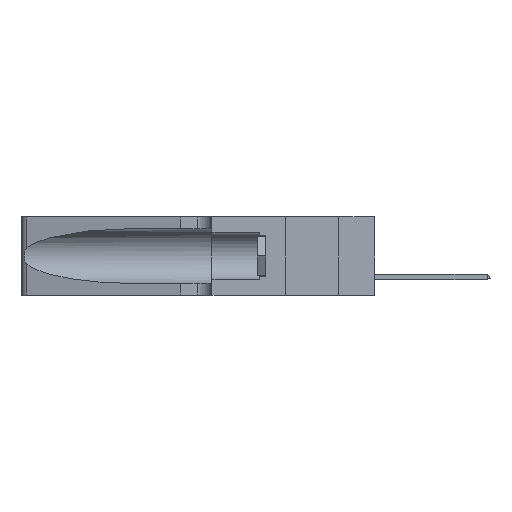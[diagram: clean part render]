
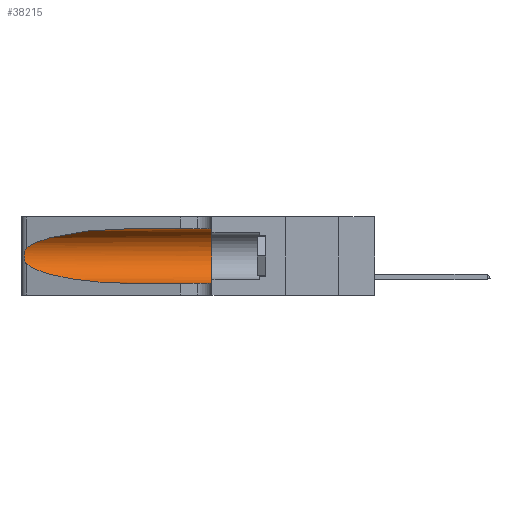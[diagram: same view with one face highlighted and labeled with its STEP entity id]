
A CAD part, left-side view. The second image highlights one B-rep face of the part: STEP entity #38215.
In plain terms, the highlighted cylindrical face has radius 3.308 mm (diameter 6.617 mm), a partial arc.
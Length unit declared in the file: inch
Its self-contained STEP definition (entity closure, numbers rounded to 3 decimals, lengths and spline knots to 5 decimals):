
#471 = DIRECTION ( 'NONE',  ( 0., 0., -1. ) ) ;
#1539 = FACE_OUTER_BOUND ( 'NONE', #27234, .T. ) ;
#2206 = CARTESIAN_POINT ( 'NONE',  ( 0.1305, 1.61858, 0.31525 ) ) ;
#2601 = CARTESIAN_POINT ( 'NONE',  ( 0.25555, 1.22993, 0.14849 ) ) ;
#4434 = EDGE_CURVE ( 'NONE', #15458, #45170, #33483, .T. ) ;
#5047 = CARTESIAN_POINT ( 'NONE',  ( 0.18966, 0.96281, 0.05475 ) ) ;
#5247 = CARTESIAN_POINT ( 'NONE',  ( 0.1305, 0.72297, 0.31525 ) ) ;
#7625 = B_SPLINE_CURVE_WITH_KNOTS ( 'NONE', 3,
 ( #9931, #10079, #45589, #45421, #24089, #35086, #41959, #20405, #34930, #30818, #23931, #38529, #2601, #17124 ),
 .UNSPECIFIED., .F., .F.,
 ( 4, 2, 2, 2, 2, 2, 4 ),
 ( 0., 0.00027, 0.00053, 0.00107, 0.0016, 0.00187, 0.00214 ),
 .UNSPECIFIED. ) ;
#8610 = CARTESIAN_POINT ( 'NONE',  ( 0.25487, 1.22718, 0.14631 ) ) ;
#8734 = DIRECTION ( 'NONE',  ( 0., -1., 0. ) ) ;
#8742 = ORIENTED_EDGE ( 'NONE', *, *, #41999, .T. ) ;
#8799 = ORIENTED_EDGE ( 'NONE', *, *, #36739, .T. ) ;
#9746 = VERTEX_POINT ( 'NONE', #41527 ) ;
#9931 = CARTESIAN_POINT ( 'NONE',  ( 0.25487, 1.22718, 0.22369 ) ) ;
#10079 = CARTESIAN_POINT ( 'NONE',  ( 0.25555, 1.22994, 0.2215 ) ) ;
#13579 = ORIENTED_EDGE ( 'NONE', *, *, #36324, .T. ) ;
#13981 = DIRECTION ( 'NONE',  ( 0., -1., 0. ) ) ;
#15458 = VERTEX_POINT ( 'NONE', #39238 ) ;
#15494 = CARTESIAN_POINT ( 'NONE',  ( 0.2373, 1.15595, 0.28018 ) ) ;
#16276 = VECTOR ( 'NONE', #19708, 39.37008 ) ;
#16308 = ORIENTED_EDGE ( 'NONE', *, *, #30351, .T. ) ;
#17124 = CARTESIAN_POINT ( 'NONE',  ( 0.25487, 1.22718, 0.14631 ) ) ;
#17730 = VERTEX_POINT ( 'NONE', #44135 ) ;
#18929 = CARTESIAN_POINT ( 'NONE',  ( 0.2373, 1.15595, 0.08982 ) ) ;
#19708 = DIRECTION ( 'NONE',  ( 0., -1., 0. ) ) ;
#20157 = VECTOR ( 'NONE', #8734, 39.37008 ) ;
#20405 = CARTESIAN_POINT ( 'NONE',  ( 0.26075, 1.23896, 0.178 ) ) ;
#22241 = CARTESIAN_POINT ( 'NONE',  ( 0.1305, 0.35, 0.185 ) ) ;
#22394 = DIRECTION ( 'NONE',  ( 0., 1., 0. ) ) ;
#22819 = CARTESIAN_POINT ( 'NONE',  ( 0.1305, 0.72297, 0.05475 ) ) ;
#23931 = CARTESIAN_POINT ( 'NONE',  ( 0.25789, 1.23486, 0.15765 ) ) ;
#24089 = CARTESIAN_POINT ( 'NONE',  ( 0.25854, 1.2359, 0.20912 ) ) ;
#25613 =( BOUNDED_CURVE ( )  B_SPLINE_CURVE ( 3, ( #5247, #44721, #15494, #26215 ),
 .UNSPECIFIED., .F., .F. ) 
 B_SPLINE_CURVE_WITH_KNOTS ( ( 4, 4 ),
 ( 1.5708, 2.84003 ),
 .UNSPECIFIED. ) 
 CURVE ( )  GEOMETRIC_REPRESENTATION_ITEM ( )  RATIONAL_B_SPLINE_CURVE ( ( 1., 0.87, 0.87, 1. ) ) 
 REPRESENTATION_ITEM ( '' )  );
#25808 = DIRECTION ( 'NONE',  ( 0., 0., 1. ) ) ;
#26215 = CARTESIAN_POINT ( 'NONE',  ( 0.25487, 1.22718, 0.22369 ) ) ;
#27201 = ORIENTED_EDGE ( 'NONE', *, *, #4434, .F. ) ;
#27234 = EDGE_LOOP ( 'NONE', ( #8799, #16308, #8742, #13579, #30897, #27201 ) ) ;
#30095 = VERTEX_POINT ( 'NONE', #37146 ) ;
#30351 = EDGE_CURVE ( 'NONE', #17730, #30095, #7625, .T. ) ;
#30818 = CARTESIAN_POINT ( 'NONE',  ( 0.25856, 1.23593, 0.16098 ) ) ;
#30823 = AXIS2_PLACEMENT_3D ( 'NONE', #22241, #22394, #25808 ) ;
#30897 = ORIENTED_EDGE ( 'NONE', *, *, #45997, .F. ) ;
#31753 = CARTESIAN_POINT ( 'NONE',  ( 0.1305, 1.61858, 0.185 ) ) ;
#31939 = CARTESIAN_POINT ( 'NONE',  ( 0.1305, 1.61858, 0.05475 ) ) ;
#32860 = CIRCLE ( 'NONE', #30823, 0.13025 ) ;
#33483 = LINE ( 'NONE', #2206, #20157 ) ;
#33571 = CARTESIAN_POINT ( 'NONE',  ( 0.1305, 0.72297, 0.05475 ) ) ;
#34930 = CARTESIAN_POINT ( 'NONE',  ( 0.26017, 1.23833, 0.17102 ) ) ;
#35086 = CARTESIAN_POINT ( 'NONE',  ( 0.26018, 1.23835, 0.19895 ) ) ;
#35220 =( BOUNDED_CURVE ( )  B_SPLINE_CURVE ( 3, ( #8610, #18929, #5047, #33571 ),
 .UNSPECIFIED., .F., .F. ) 
 B_SPLINE_CURVE_WITH_KNOTS ( ( 4, 4 ),
 ( 3.44316, 4.71239 ),
 .UNSPECIFIED. ) 
 CURVE ( )  GEOMETRIC_REPRESENTATION_ITEM ( )  RATIONAL_B_SPLINE_CURVE ( ( 1., 0.87, 0.87, 1. ) ) 
 REPRESENTATION_ITEM ( '' )  );
#35318 = LINE ( 'NONE', #31939, #16276 ) ;
#36324 = EDGE_CURVE ( 'NONE', #36533, #9746, #35318, .T. ) ;
#36533 = VERTEX_POINT ( 'NONE', #22819 ) ;
#36739 = EDGE_CURVE ( 'NONE', #15458, #17730, #25613, .T. ) ;
#37146 = CARTESIAN_POINT ( 'NONE',  ( 0.25487, 1.22718, 0.14631 ) ) ;
#37841 = CYLINDRICAL_SURFACE ( 'NONE', #42664, 0.13025 ) ;
#38215 = ADVANCED_FACE ( 'NONE', ( #1539 ), #37841, .F. ) ;
#38529 = CARTESIAN_POINT ( 'NONE',  ( 0.25639, 1.23186, 0.15144 ) ) ;
#39238 = CARTESIAN_POINT ( 'NONE',  ( 0.1305, 0.72297, 0.31525 ) ) ;
#39422 = CARTESIAN_POINT ( 'NONE',  ( 0.1305, 0.35, 0.31525 ) ) ;
#41527 = CARTESIAN_POINT ( 'NONE',  ( 0.1305, 0.35, 0.05475 ) ) ;
#41959 = CARTESIAN_POINT ( 'NONE',  ( 0.26075, 1.23896, 0.19203 ) ) ;
#41999 = EDGE_CURVE ( 'NONE', #30095, #36533, #35220, .T. ) ;
#42664 = AXIS2_PLACEMENT_3D ( 'NONE', #31753, #13981, #471 ) ;
#44135 = CARTESIAN_POINT ( 'NONE',  ( 0.25487, 1.22718, 0.22369 ) ) ;
#44721 = CARTESIAN_POINT ( 'NONE',  ( 0.18966, 0.96281, 0.31525 ) ) ;
#45170 = VERTEX_POINT ( 'NONE', #39422 ) ;
#45421 = CARTESIAN_POINT ( 'NONE',  ( 0.25787, 1.23484, 0.2124 ) ) ;
#45589 = CARTESIAN_POINT ( 'NONE',  ( 0.25639, 1.23184, 0.21858 ) ) ;
#45997 = EDGE_CURVE ( 'NONE', #45170, #9746, #32860, .T. ) ;
